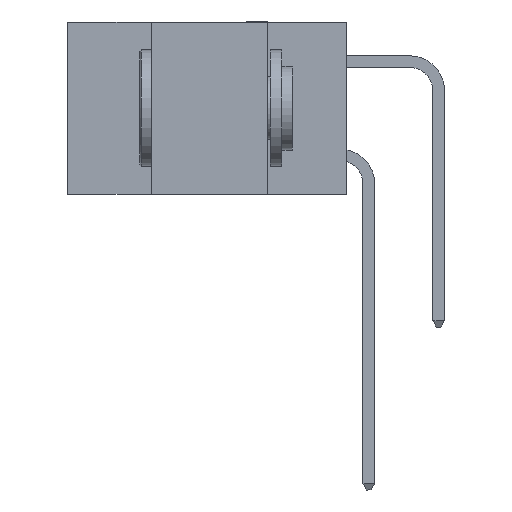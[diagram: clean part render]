
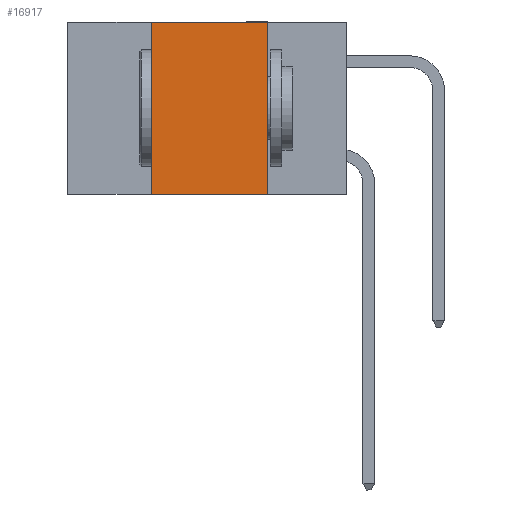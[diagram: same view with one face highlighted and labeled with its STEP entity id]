
A CAD part, left-side view. The second image highlights one B-rep face of the part: STEP entity #16917.
In plain terms, the highlighted planar face has unit normal (-1, 0, 0).
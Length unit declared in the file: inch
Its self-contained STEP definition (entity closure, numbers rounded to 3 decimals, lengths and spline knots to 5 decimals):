
#167 = ORIENTED_EDGE ( 'NONE', *, *, #1873, .T. ) ;
#282 = PLANE ( 'NONE',  #1341 ) ;
#679 = LINE ( 'NONE', #2135, #9545 ) ;
#1341 = AXIS2_PLACEMENT_3D ( 'NONE', #3559, #14309, #5168 ) ;
#1468 = EDGE_CURVE ( 'NONE', #16397, #16350, #679, .T. ) ;
#1873 = EDGE_CURVE ( 'NONE', #16397, #19297, #3878, .T. ) ;
#2135 = CARTESIAN_POINT ( 'NONE',  ( 0., 0.42, 0. ) ) ;
#2159 = DIRECTION ( 'NONE',  ( 0., 0., 1. ) ) ;
#2412 = ORIENTED_EDGE ( 'NONE', *, *, #12904, .F. ) ;
#3559 = CARTESIAN_POINT ( 'NONE',  ( 0., 0.6, 0. ) ) ;
#3878 = LINE ( 'NONE', #19758, #19527 ) ;
#5034 = FACE_OUTER_BOUND ( 'NONE', #19377, .T. ) ;
#5168 = DIRECTION ( 'NONE',  ( 0., 0., -1. ) ) ;
#5395 = ORIENTED_EDGE ( 'NONE', *, *, #18797, .F. ) ;
#6174 = ORIENTED_EDGE ( 'NONE', *, *, #1468, .F. ) ;
#6696 = DIRECTION ( 'NONE',  ( 0., -1., 0. ) ) ;
#9545 = VECTOR ( 'NONE', #2159, 39.37008 ) ;
#10405 = CARTESIAN_POINT ( 'NONE',  ( 0., 0.17, 0. ) ) ;
#11658 = CARTESIAN_POINT ( 'NONE',  ( 0., 0.42, 0. ) ) ;
#11792 = LINE ( 'NONE', #10405, #14765 ) ;
#12734 = CARTESIAN_POINT ( 'NONE',  ( 0., 0.6, 0. ) ) ;
#12904 = EDGE_CURVE ( 'NONE', #17702, #19297, #11792, .T. ) ;
#14309 = DIRECTION ( 'NONE',  ( 1., 0., 0. ) ) ;
#14765 = VECTOR ( 'NONE', #19259, 39.37008 ) ;
#14875 = VECTOR ( 'NONE', #6696, 39.37008 ) ;
#15338 = LINE ( 'NONE', #12734, #14875 ) ;
#16350 = VERTEX_POINT ( 'NONE', #11658 ) ;
#16397 = VERTEX_POINT ( 'NONE', #19091 ) ;
#16917 = ADVANCED_FACE ( 'NONE', ( #5034 ), #282, .F. ) ;
#17702 = VERTEX_POINT ( 'NONE', #17868 ) ;
#17868 = CARTESIAN_POINT ( 'NONE',  ( 0., 0.17, 0. ) ) ;
#18575 = CARTESIAN_POINT ( 'NONE',  ( 0., 0.17, -0.37 ) ) ;
#18797 = EDGE_CURVE ( 'NONE', #16350, #17702, #15338, .T. ) ;
#19091 = CARTESIAN_POINT ( 'NONE',  ( 0., 0.42, -0.37 ) ) ;
#19259 = DIRECTION ( 'NONE',  ( 0., 0., -1. ) ) ;
#19297 = VERTEX_POINT ( 'NONE', #18575 ) ;
#19377 = EDGE_LOOP ( 'NONE', ( #2412, #5395, #6174, #167 ) ) ;
#19527 = VECTOR ( 'NONE', #19583, 39.37008 ) ;
#19583 = DIRECTION ( 'NONE',  ( 0., -1., 0. ) ) ;
#19758 = CARTESIAN_POINT ( 'NONE',  ( 0., 0.6, -0.37 ) ) ;
